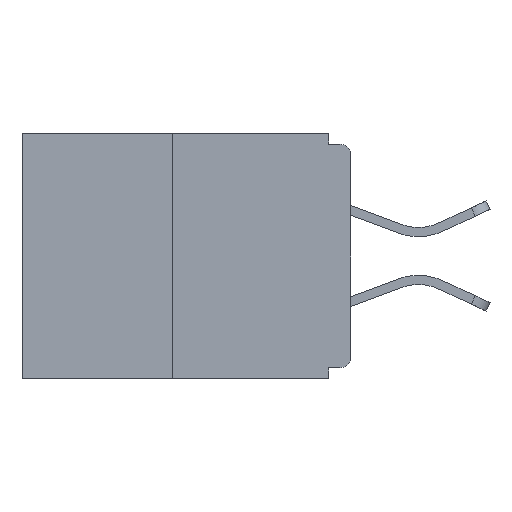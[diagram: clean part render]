
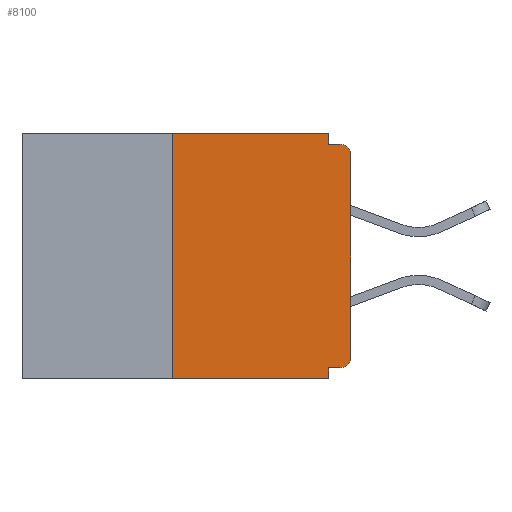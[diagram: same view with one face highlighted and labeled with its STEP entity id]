
A CAD part, left-side view. The second image highlights one B-rep face of the part: STEP entity #8100.
In plain terms, the highlighted planar face has unit normal (-1, 0, 0).
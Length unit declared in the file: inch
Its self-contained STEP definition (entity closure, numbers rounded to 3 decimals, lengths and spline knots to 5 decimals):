
#243 = DIRECTION ( 'NONE',  ( 0., 0., 1. ) ) ;
#319 = CARTESIAN_POINT ( 'NONE',  ( 0., 0.031, -0.343 ) ) ;
#509 = EDGE_LOOP ( 'NONE', ( #17010, #3222, #15131, #1583, #15031, #11289, #12990, #10526, #10663, #13930 ) ) ;
#768 = CARTESIAN_POINT ( 'NONE',  ( 0., 0.015, -0.313 ) ) ;
#999 = CARTESIAN_POINT ( 'NONE',  ( 0., 0.25, -0.343 ) ) ;
#1583 = ORIENTED_EDGE ( 'NONE', *, *, #19683, .F. ) ;
#1872 = VERTEX_POINT ( 'NONE', #9505 ) ;
#1950 = VERTEX_POINT ( 'NONE', #999 ) ;
#2444 = VECTOR ( 'NONE', #243, 39.37008 ) ;
#2523 = VECTOR ( 'NONE', #5951, 39.37008 ) ;
#2576 = LINE ( 'NONE', #3554, #22362 ) ;
#2652 = VECTOR ( 'NONE', #15779, 39.37008 ) ;
#2891 = CARTESIAN_POINT ( 'NONE',  ( 0., 0.015, -0.328 ) ) ;
#3222 = ORIENTED_EDGE ( 'NONE', *, *, #22609, .F. ) ;
#3517 = VECTOR ( 'NONE', #7866, 39.37008 ) ;
#3554 = CARTESIAN_POINT ( 'NONE',  ( 0., 0.25, 0. ) ) ;
#3645 = AXIS2_PLACEMENT_3D ( 'NONE', #22341, #20439, #8240 ) ;
#4161 = CIRCLE ( 'NONE', #5946, 0.015 ) ;
#4189 = DIRECTION ( 'NONE',  ( -1., 0., 0. ) ) ;
#4597 = LINE ( 'NONE', #13970, #2652 ) ;
#4635 = LINE ( 'NONE', #6072, #3517 ) ;
#4845 = EDGE_CURVE ( 'NONE', #15293, #1872, #6326, .T. ) ;
#5099 = LINE ( 'NONE', #11661, #18761 ) ;
#5213 = LINE ( 'NONE', #319, #6570 ) ;
#5946 = AXIS2_PLACEMENT_3D ( 'NONE', #768, #4189, #18436 ) ;
#5951 = DIRECTION ( 'NONE',  ( 0., -1., 0. ) ) ;
#5959 = DIRECTION ( 'NONE',  ( 1., 0., 0. ) ) ;
#6072 = CARTESIAN_POINT ( 'NONE',  ( 0., 0., -0.015 ) ) ;
#6326 = LINE ( 'NONE', #17463, #22221 ) ;
#6570 = VECTOR ( 'NONE', #12761, 39.37008 ) ;
#7196 = EDGE_CURVE ( 'NONE', #21808, #17980, #15884, .T. ) ;
#7688 = PLANE ( 'NONE',  #22525 ) ;
#7866 = DIRECTION ( 'NONE',  ( 0., -1., 0. ) ) ;
#7886 = DIRECTION ( 'NONE',  ( 0., 0., -1. ) ) ;
#7997 = CARTESIAN_POINT ( 'NONE',  ( 0., 0.015, -0.015 ) ) ;
#8053 = CARTESIAN_POINT ( 'NONE',  ( 0., 0.25, 0. ) ) ;
#8100 = ADVANCED_FACE ( 'NONE', ( #22244 ), #7688, .F. ) ;
#8191 = CARTESIAN_POINT ( 'NONE',  ( 0., 0.031, 0. ) ) ;
#8240 = DIRECTION ( 'NONE',  ( 0., 0., -1. ) ) ;
#9505 = CARTESIAN_POINT ( 'NONE',  ( 0., 0.031, -0.328 ) ) ;
#10526 = ORIENTED_EDGE ( 'NONE', *, *, #12391, .T. ) ;
#10663 = ORIENTED_EDGE ( 'NONE', *, *, #17045, .F. ) ;
#11289 = ORIENTED_EDGE ( 'NONE', *, *, #15188, .T. ) ;
#11396 = CARTESIAN_POINT ( 'NONE',  ( 0., 0.46, 0. ) ) ;
#11661 = CARTESIAN_POINT ( 'NONE',  ( 0., 0.031, 0. ) ) ;
#12362 = DIRECTION ( 'NONE',  ( 0., 0., 1. ) ) ;
#12391 = EDGE_CURVE ( 'NONE', #16873, #19790, #21804, .T. ) ;
#12761 = DIRECTION ( 'NONE',  ( 0., 0., -1. ) ) ;
#12990 = ORIENTED_EDGE ( 'NONE', *, *, #19530, .T. ) ;
#13476 = CARTESIAN_POINT ( 'NONE',  ( 0., 0.031, -0.343 ) ) ;
#13930 = ORIENTED_EDGE ( 'NONE', *, *, #22371, .F. ) ;
#13970 = CARTESIAN_POINT ( 'NONE',  ( 0., 0.46, -0.343 ) ) ;
#14352 = VERTEX_POINT ( 'NONE', #13476 ) ;
#14385 = CARTESIAN_POINT ( 'NONE',  ( 0., 0., -0.03 ) ) ;
#14826 = DIRECTION ( 'NONE',  ( 0., 0., -1. ) ) ;
#14877 = CARTESIAN_POINT ( 'NONE',  ( 0., 0., -0.313 ) ) ;
#15031 = ORIENTED_EDGE ( 'NONE', *, *, #4845, .F. ) ;
#15131 = ORIENTED_EDGE ( 'NONE', *, *, #17655, .T. ) ;
#15188 = EDGE_CURVE ( 'NONE', #15293, #22233, #4161, .T. ) ;
#15287 = VERTEX_POINT ( 'NONE', #16953 ) ;
#15293 = VERTEX_POINT ( 'NONE', #2891 ) ;
#15754 = DIRECTION ( 'NONE',  ( 0., 1., 0. ) ) ;
#15779 = DIRECTION ( 'NONE',  ( 0., -1., 0. ) ) ;
#15884 = LINE ( 'NONE', #18109, #2523 ) ;
#16873 = VERTEX_POINT ( 'NONE', #14385 ) ;
#16953 = CARTESIAN_POINT ( 'NONE',  ( 0., 0.031, -0.015 ) ) ;
#17010 = ORIENTED_EDGE ( 'NONE', *, *, #7196, .F. ) ;
#17045 = EDGE_CURVE ( 'NONE', #15287, #19790, #4635, .T. ) ;
#17463 = CARTESIAN_POINT ( 'NONE',  ( 0., 0., -0.328 ) ) ;
#17655 = EDGE_CURVE ( 'NONE', #1950, #14352, #4597, .T. ) ;
#17980 = VERTEX_POINT ( 'NONE', #8191 ) ;
#18109 = CARTESIAN_POINT ( 'NONE',  ( 0., 0.46, 0. ) ) ;
#18436 = DIRECTION ( 'NONE',  ( 0., 0., -1. ) ) ;
#18761 = VECTOR ( 'NONE', #7886, 39.37008 ) ;
#18872 = LINE ( 'NONE', #19641, #2444 ) ;
#19530 = EDGE_CURVE ( 'NONE', #22233, #16873, #18872, .T. ) ;
#19641 = CARTESIAN_POINT ( 'NONE',  ( 0., 0., 0. ) ) ;
#19683 = EDGE_CURVE ( 'NONE', #1872, #14352, #5213, .T. ) ;
#19790 = VERTEX_POINT ( 'NONE', #7997 ) ;
#20439 = DIRECTION ( 'NONE',  ( -1., 0., 0. ) ) ;
#21804 = CIRCLE ( 'NONE', #3645, 0.015 ) ;
#21808 = VERTEX_POINT ( 'NONE', #8053 ) ;
#22221 = VECTOR ( 'NONE', #15754, 39.37008 ) ;
#22233 = VERTEX_POINT ( 'NONE', #14877 ) ;
#22244 = FACE_OUTER_BOUND ( 'NONE', #509, .T. ) ;
#22341 = CARTESIAN_POINT ( 'NONE',  ( 0., 0.015, -0.03 ) ) ;
#22362 = VECTOR ( 'NONE', #12362, 39.37008 ) ;
#22371 = EDGE_CURVE ( 'NONE', #17980, #15287, #5099, .T. ) ;
#22525 = AXIS2_PLACEMENT_3D ( 'NONE', #11396, #5959, #14826 ) ;
#22609 = EDGE_CURVE ( 'NONE', #1950, #21808, #2576, .T. ) ;
